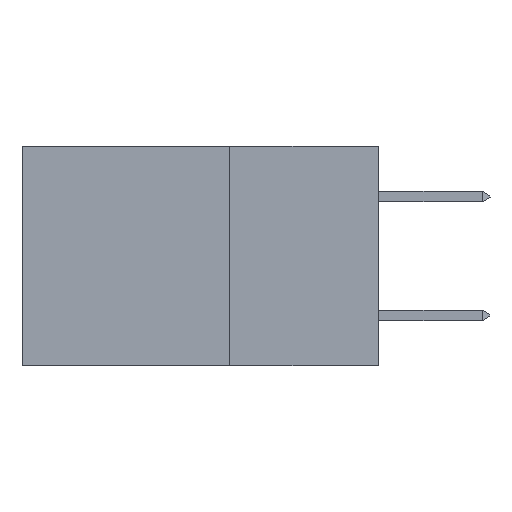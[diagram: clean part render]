
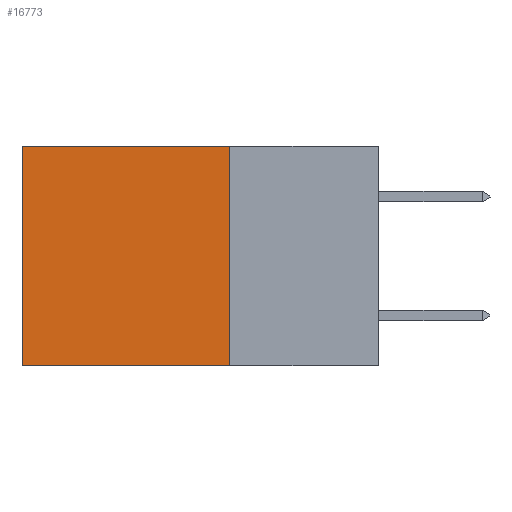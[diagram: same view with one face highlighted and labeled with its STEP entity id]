
A CAD part, left-side view. The second image highlights one B-rep face of the part: STEP entity #16773.
In plain terms, the highlighted planar face has unit normal (-1, 0, 0).
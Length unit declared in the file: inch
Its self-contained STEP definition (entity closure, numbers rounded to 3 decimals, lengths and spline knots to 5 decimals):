
#122 = CARTESIAN_POINT ( 'NONE',  ( 0.298, 0.25, 0. ) ) ;
#146 = CARTESIAN_POINT ( 'NONE',  ( 0.298, 0.25, 0. ) ) ;
#536 = EDGE_CURVE ( 'NONE', #3607, #4424, #17366, .T. ) ;
#1337 = LINE ( 'NONE', #16356, #17640 ) ;
#1729 = VECTOR ( 'NONE', #3037, 39.37008 ) ;
#3037 = DIRECTION ( 'NONE',  ( 0., 0., -1. ) ) ;
#3607 = VERTEX_POINT ( 'NONE', #7666 ) ;
#4071 = LINE ( 'NONE', #15531, #1729 ) ;
#4424 = VERTEX_POINT ( 'NONE', #18415 ) ;
#4545 = AXIS2_PLACEMENT_3D ( 'NONE', #122, #16992, #13567 ) ;
#5175 = EDGE_CURVE ( 'NONE', #9286, #3607, #12116, .T. ) ;
#5606 = EDGE_CURVE ( 'NONE', #9286, #7411, #4071, .T. ) ;
#7411 = VERTEX_POINT ( 'NONE', #8489 ) ;
#7666 = CARTESIAN_POINT ( 'NONE',  ( 0.298, 0.6, 0. ) ) ;
#7919 = VECTOR ( 'NONE', #11845, 39.37008 ) ;
#8489 = CARTESIAN_POINT ( 'NONE',  ( 0.298, 0.25, -0.37 ) ) ;
#8775 = ORIENTED_EDGE ( 'NONE', *, *, #536, .T. ) ;
#8879 = EDGE_LOOP ( 'NONE', ( #8775, #10629, #10977, #10006 ) ) ;
#9286 = VERTEX_POINT ( 'NONE', #146 ) ;
#10006 = ORIENTED_EDGE ( 'NONE', *, *, #5175, .T. ) ;
#10629 = ORIENTED_EDGE ( 'NONE', *, *, #22791, .F. ) ;
#10752 = CARTESIAN_POINT ( 'NONE',  ( 0.298, 0.25, 0. ) ) ;
#10908 = DIRECTION ( 'NONE',  ( 0., 1., 0. ) ) ;
#10977 = ORIENTED_EDGE ( 'NONE', *, *, #5606, .F. ) ;
#11845 = DIRECTION ( 'NONE',  ( 0., 0., -1. ) ) ;
#12116 = LINE ( 'NONE', #10752, #21268 ) ;
#13567 = DIRECTION ( 'NONE',  ( 0., 0., -1. ) ) ;
#15531 = CARTESIAN_POINT ( 'NONE',  ( 0.298, 0.25, 0. ) ) ;
#16356 = CARTESIAN_POINT ( 'NONE',  ( 0.298, 0.25, -0.37 ) ) ;
#16773 = ADVANCED_FACE ( 'NONE', ( #21324 ), #22017, .F. ) ;
#16992 = DIRECTION ( 'NONE',  ( 1., 0., 0. ) ) ;
#17362 = CARTESIAN_POINT ( 'NONE',  ( 0.298, 0.6, 0. ) ) ;
#17366 = LINE ( 'NONE', #17362, #7919 ) ;
#17640 = VECTOR ( 'NONE', #10908, 39.37008 ) ;
#18415 = CARTESIAN_POINT ( 'NONE',  ( 0.298, 0.6, -0.37 ) ) ;
#21268 = VECTOR ( 'NONE', #21715, 39.37008 ) ;
#21324 = FACE_OUTER_BOUND ( 'NONE', #8879, .T. ) ;
#21715 = DIRECTION ( 'NONE',  ( 0., 1., 0. ) ) ;
#22017 = PLANE ( 'NONE',  #4545 ) ;
#22791 = EDGE_CURVE ( 'NONE', #7411, #4424, #1337, .T. ) ;
